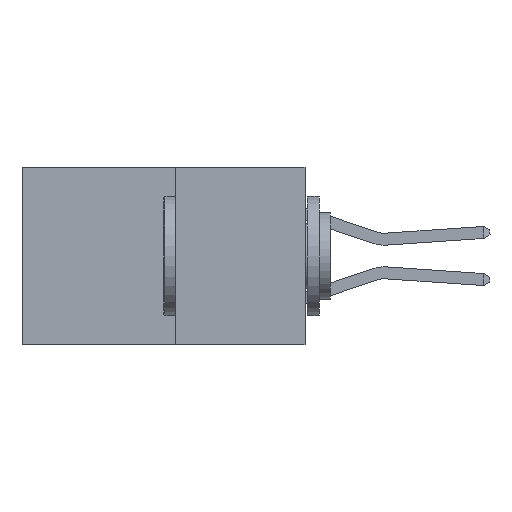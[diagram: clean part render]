
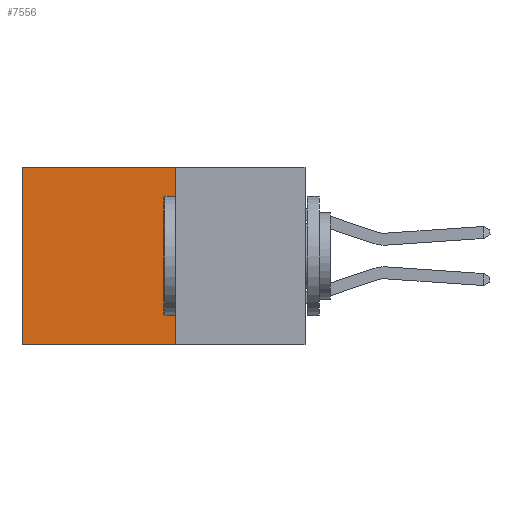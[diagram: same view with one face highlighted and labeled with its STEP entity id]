
A CAD part, left-side view. The second image highlights one B-rep face of the part: STEP entity #7556.
In plain terms, the highlighted planar face has unit normal (-1, 0, 0).
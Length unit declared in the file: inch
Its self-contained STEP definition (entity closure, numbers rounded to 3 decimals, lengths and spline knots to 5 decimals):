
#2384 = FACE_OUTER_BOUND ( 'NONE', #13822, .T. ) ;
#2844 = VECTOR ( 'NONE', #11723, 39.37008 ) ;
#5624 = VECTOR ( 'NONE', #13176, 39.37008 ) ;
#6347 = EDGE_CURVE ( 'NONE', #10396, #26712, #22356, .T. ) ;
#7542 = LINE ( 'NONE', #20428, #26807 ) ;
#7556 = ADVANCED_FACE ( 'NONE', ( #2384 ), #20093, .F. ) ;
#8258 = DIRECTION ( 'NONE',  ( 0., 1., 0. ) ) ;
#10396 = VERTEX_POINT ( 'NONE', #29829 ) ;
#10723 = CARTESIAN_POINT ( 'NONE',  ( 0.277, 0.59, -0.37 ) ) ;
#11723 = DIRECTION ( 'NONE',  ( 0., 1., 0. ) ) ;
#11831 = CARTESIAN_POINT ( 'NONE',  ( 0.277, 0.27, -0.37 ) ) ;
#13088 = CARTESIAN_POINT ( 'NONE',  ( 0.277, 0.59, 0. ) ) ;
#13176 = DIRECTION ( 'NONE',  ( 0., 0., -1. ) ) ;
#13323 = VERTEX_POINT ( 'NONE', #13429 ) ;
#13429 = CARTESIAN_POINT ( 'NONE',  ( 0.277, 0.27, 0. ) ) ;
#13744 = CARTESIAN_POINT ( 'NONE',  ( 0.277, 0.59, -0.37 ) ) ;
#13822 = EDGE_LOOP ( 'NONE', ( #28237, #17913, #25150, #21825 ) ) ;
#13928 = EDGE_CURVE ( 'NONE', #16520, #26712, #30442, .T. ) ;
#14012 = VECTOR ( 'NONE', #14202, 39.37008 ) ;
#14202 = DIRECTION ( 'NONE',  ( 0., 0., -1. ) ) ;
#14458 = AXIS2_PLACEMENT_3D ( 'NONE', #20590, #19921, #19824 ) ;
#15967 = EDGE_CURVE ( 'NONE', #13323, #16520, #7542, .T. ) ;
#16520 = VERTEX_POINT ( 'NONE', #13088 ) ;
#17606 = EDGE_CURVE ( 'NONE', #13323, #10396, #20470, .T. ) ;
#17913 = ORIENTED_EDGE ( 'NONE', *, *, #6347, .F. ) ;
#19824 = DIRECTION ( 'NONE',  ( 0., 0., -1. ) ) ;
#19921 = DIRECTION ( 'NONE',  ( 1., 0., 0. ) ) ;
#20093 = PLANE ( 'NONE',  #14458 ) ;
#20428 = CARTESIAN_POINT ( 'NONE',  ( 0.277, 0.27, 0. ) ) ;
#20470 = LINE ( 'NONE', #26034, #14012 ) ;
#20590 = CARTESIAN_POINT ( 'NONE',  ( 0.277, 0.27, -0.37 ) ) ;
#21825 = ORIENTED_EDGE ( 'NONE', *, *, #15967, .T. ) ;
#22356 = LINE ( 'NONE', #11831, #2844 ) ;
#25150 = ORIENTED_EDGE ( 'NONE', *, *, #17606, .F. ) ;
#26034 = CARTESIAN_POINT ( 'NONE',  ( 0.277, 0.27, -0.37 ) ) ;
#26712 = VERTEX_POINT ( 'NONE', #13744 ) ;
#26807 = VECTOR ( 'NONE', #8258, 39.37008 ) ;
#28237 = ORIENTED_EDGE ( 'NONE', *, *, #13928, .T. ) ;
#29829 = CARTESIAN_POINT ( 'NONE',  ( 0.277, 0.27, -0.37 ) ) ;
#30442 = LINE ( 'NONE', #10723, #5624 ) ;
